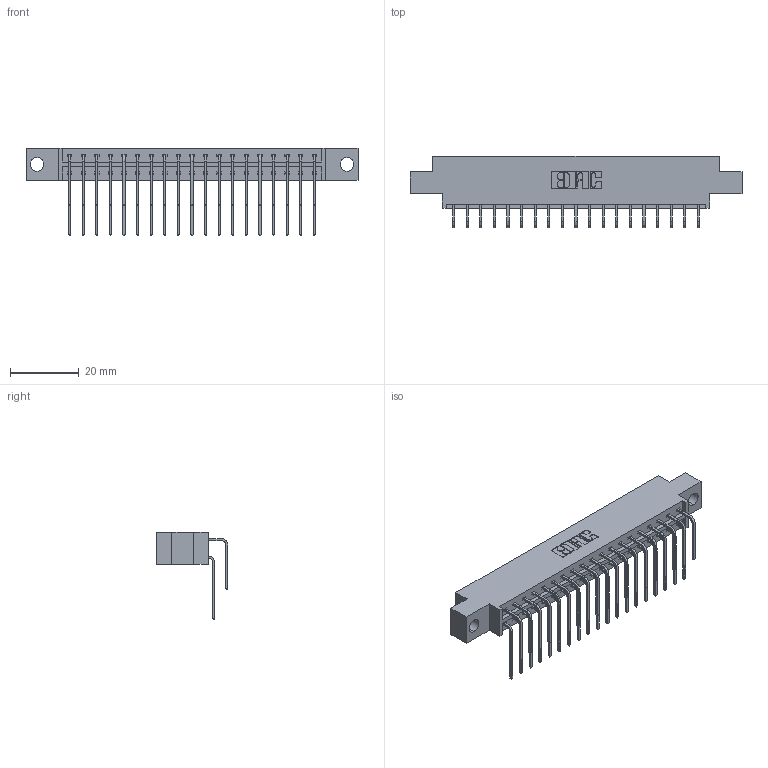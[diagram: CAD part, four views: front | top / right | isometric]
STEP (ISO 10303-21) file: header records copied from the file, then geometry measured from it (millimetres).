
FILE_DESCRIPTION (( 'STEP AP203' ), '1' );
FILE_NAME ('833-038-559-804.STEP', '2020-06-03T14:00:22', ( '' ), ( '' ), 'SwSTEP 2.0', 'SolidWorks 2020', '' );
FILE_SCHEMA (( 'CONFIG_CONTROL_DESIGN' ));
Length unit declared in the file: inch
Products named in the file (4): 833 Part_Offset - .156 Dia - TH; 833-038-559-804; 345-292-001_558 559 Tail - 1; 345-292-001_559 Tail - 2
Assembly tree (39 placements, depth 2):
  833-038-559-804
    833 Part_Offset - .156 Dia - TH
    345-292-001_558 559 Tail - 1  x19
    345-292-001_559 Tail - 2  x19
Bounding box: 96.82 x 20.9 x 25.53 mm (x, y, z)
Volume: 9573.7 mm3; surface area: 12183.5 mm2
Topology: 39 solids, 39 shells, 2170 faces, 6441 edges, 4242 vertices
Faces by surface type: plane 1518, cylinder 652
Entity records: 17117 total; most frequent: CARTESIAN_POINT 2917, ORIENTED_EDGE 2802, DIRECTION 2513, EDGE_CURVE 1401, VECTOR 1233, LINE 1233, VERTEX_POINT 930, AXIS2_PLACEMENT_3D 640
